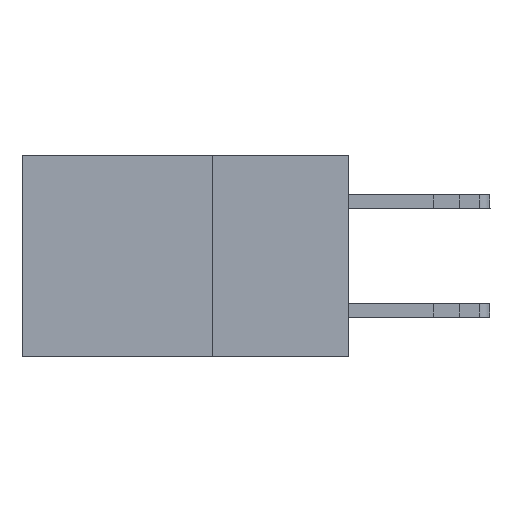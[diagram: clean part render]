
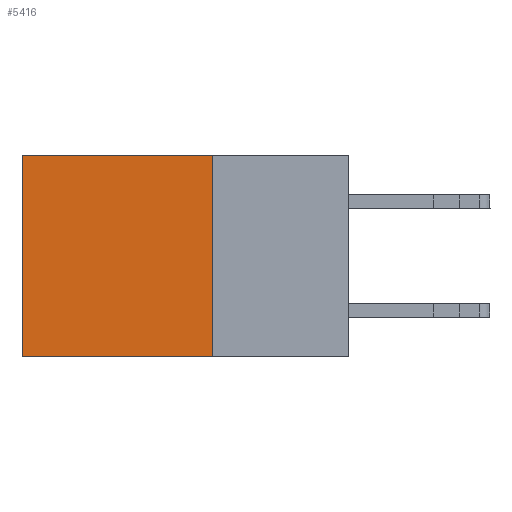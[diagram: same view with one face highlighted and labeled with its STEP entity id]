
A CAD part, left-side view. The second image highlights one B-rep face of the part: STEP entity #5416.
In plain terms, the highlighted planar face has unit normal (-1, 0, 0).
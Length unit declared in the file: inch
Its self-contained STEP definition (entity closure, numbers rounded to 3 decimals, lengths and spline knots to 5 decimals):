
#404 = PLANE ( 'NONE',  #3021 ) ;
#524 = CARTESIAN_POINT ( 'NONE',  ( 0.2615, 0.25, -0.37 ) ) ;
#909 = CARTESIAN_POINT ( 'NONE',  ( 0.2615, 0.6, -0.37 ) ) ;
#2791 = CARTESIAN_POINT ( 'NONE',  ( 0.2615, 0.25, 0. ) ) ;
#3021 = AXIS2_PLACEMENT_3D ( 'NONE', #6824, #3255, #11881 ) ;
#3145 = DIRECTION ( 'NONE',  ( 0., 0., -1. ) ) ;
#3255 = DIRECTION ( 'NONE',  ( 1., 0., 0. ) ) ;
#3369 = VERTEX_POINT ( 'NONE', #9663 ) ;
#3661 = CARTESIAN_POINT ( 'NONE',  ( 0.2615, 0.25, 0. ) ) ;
#5337 = VERTEX_POINT ( 'NONE', #2791 ) ;
#5402 = LINE ( 'NONE', #524, #6788 ) ;
#5416 = ADVANCED_FACE ( 'NONE', ( #11960 ), #404, .F. ) ;
#5614 = EDGE_CURVE ( 'NONE', #13055, #16146, #9781, .T. ) ;
#6315 = LINE ( 'NONE', #3661, #15746 ) ;
#6788 = VECTOR ( 'NONE', #9194, 39.37008 ) ;
#6824 = CARTESIAN_POINT ( 'NONE',  ( 0.2615, 0.25, -0.37 ) ) ;
#8550 = DIRECTION ( 'NONE',  ( 0., 1., 0. ) ) ;
#8927 = EDGE_CURVE ( 'NONE', #3369, #16146, #15997, .T. ) ;
#9047 = CARTESIAN_POINT ( 'NONE',  ( 0.2615, 0.25, -0.37 ) ) ;
#9194 = DIRECTION ( 'NONE',  ( 0., 0., -1. ) ) ;
#9218 = EDGE_LOOP ( 'NONE', ( #11778, #12011, #13930, #15382 ) ) ;
#9663 = CARTESIAN_POINT ( 'NONE',  ( 0.2615, 0.6, 0. ) ) ;
#9781 = LINE ( 'NONE', #13621, #15743 ) ;
#9855 = DIRECTION ( 'NONE',  ( 0., 1., 0. ) ) ;
#10214 = EDGE_CURVE ( 'NONE', #5337, #13055, #5402, .T. ) ;
#10775 = VECTOR ( 'NONE', #3145, 39.37008 ) ;
#11778 = ORIENTED_EDGE ( 'NONE', *, *, #8927, .T. ) ;
#11845 = CARTESIAN_POINT ( 'NONE',  ( 0.2615, 0.6, -0.37 ) ) ;
#11881 = DIRECTION ( 'NONE',  ( 0., 0., -1. ) ) ;
#11960 = FACE_OUTER_BOUND ( 'NONE', #9218, .T. ) ;
#12011 = ORIENTED_EDGE ( 'NONE', *, *, #5614, .F. ) ;
#13055 = VERTEX_POINT ( 'NONE', #9047 ) ;
#13621 = CARTESIAN_POINT ( 'NONE',  ( 0.2615, 0.25, -0.37 ) ) ;
#13930 = ORIENTED_EDGE ( 'NONE', *, *, #10214, .F. ) ;
#15237 = EDGE_CURVE ( 'NONE', #5337, #3369, #6315, .T. ) ;
#15382 = ORIENTED_EDGE ( 'NONE', *, *, #15237, .T. ) ;
#15743 = VECTOR ( 'NONE', #8550, 39.37008 ) ;
#15746 = VECTOR ( 'NONE', #9855, 39.37008 ) ;
#15997 = LINE ( 'NONE', #11845, #10775 ) ;
#16146 = VERTEX_POINT ( 'NONE', #909 ) ;
